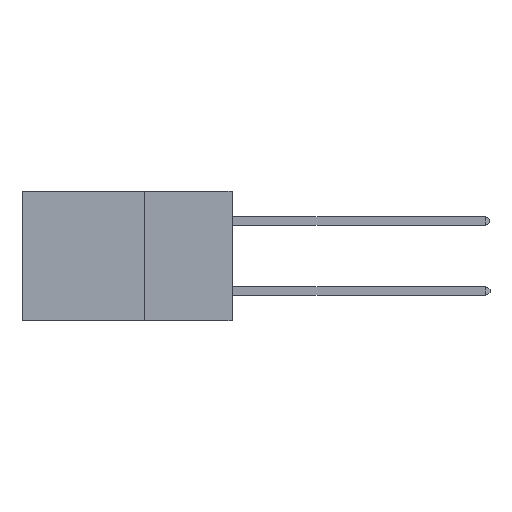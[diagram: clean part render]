
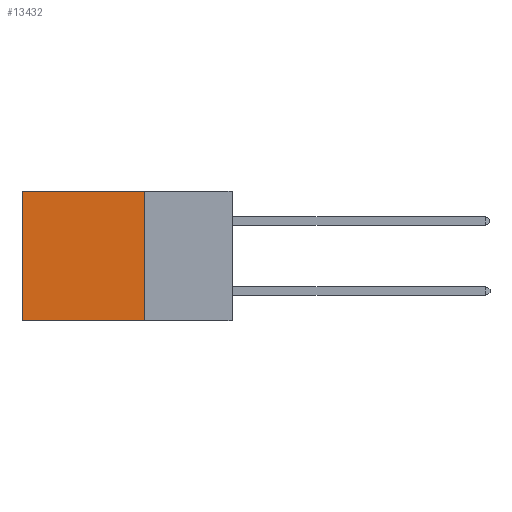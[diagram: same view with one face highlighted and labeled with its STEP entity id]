
A CAD part, left-side view. The second image highlights one B-rep face of the part: STEP entity #13432.
In plain terms, the highlighted planar face has unit normal (-1, 0, 0).
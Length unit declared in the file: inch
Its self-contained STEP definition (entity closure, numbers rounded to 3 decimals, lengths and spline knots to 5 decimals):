
#183 = CARTESIAN_POINT ( 'NONE',  ( 0.2875, 0.25, 0. ) ) ;
#424 = VECTOR ( 'NONE', #9769, 39.37008 ) ;
#2208 = CARTESIAN_POINT ( 'NONE',  ( 0.2875, 0.25, 0. ) ) ;
#2341 = VECTOR ( 'NONE', #15255, 39.37008 ) ;
#2684 = EDGE_LOOP ( 'NONE', ( #14971, #14897, #14915, #9930 ) ) ;
#2912 = EDGE_CURVE ( 'NONE', #13788, #10563, #7485, .T. ) ;
#3973 = CARTESIAN_POINT ( 'NONE',  ( 0.2875, 0.25, 0. ) ) ;
#4013 = FACE_OUTER_BOUND ( 'NONE', #2684, .T. ) ;
#4125 = CARTESIAN_POINT ( 'NONE',  ( 0.2875, 0.25, -0.37 ) ) ;
#4791 = VECTOR ( 'NONE', #8183, 39.37008 ) ;
#4951 = CARTESIAN_POINT ( 'NONE',  ( 0.2875, 0.25, -0.37 ) ) ;
#6215 = CARTESIAN_POINT ( 'NONE',  ( 0.2875, 0.25, 0. ) ) ;
#6250 = LINE ( 'NONE', #4951, #2341 ) ;
#6834 = LINE ( 'NONE', #2208, #9957 ) ;
#7485 = LINE ( 'NONE', #9855, #424 ) ;
#7552 = DIRECTION ( 'NONE',  ( 1., 0., 0. ) ) ;
#8183 = DIRECTION ( 'NONE',  ( 0., 0., -1. ) ) ;
#8412 = EDGE_CURVE ( 'NONE', #15475, #15581, #14348, .T. ) ;
#9769 = DIRECTION ( 'NONE',  ( 0., 0., -1. ) ) ;
#9855 = CARTESIAN_POINT ( 'NONE',  ( 0.2875, 0.6, 0. ) ) ;
#9929 = CARTESIAN_POINT ( 'NONE',  ( 0.2875, 0.6, -0.37 ) ) ;
#9930 = ORIENTED_EDGE ( 'NONE', *, *, #14406, .T. ) ;
#9957 = VECTOR ( 'NONE', #10134, 39.37008 ) ;
#10051 = AXIS2_PLACEMENT_3D ( 'NONE', #6215, #7552, #16421 ) ;
#10134 = DIRECTION ( 'NONE',  ( 0., 1., 0. ) ) ;
#10563 = VERTEX_POINT ( 'NONE', #9929 ) ;
#13432 = ADVANCED_FACE ( 'NONE', ( #4013 ), #14000, .F. ) ;
#13456 = EDGE_CURVE ( 'NONE', #15581, #10563, #6250, .T. ) ;
#13572 = CARTESIAN_POINT ( 'NONE',  ( 0.2875, 0.6, 0. ) ) ;
#13788 = VERTEX_POINT ( 'NONE', #13572 ) ;
#14000 = PLANE ( 'NONE',  #10051 ) ;
#14348 = LINE ( 'NONE', #183, #4791 ) ;
#14406 = EDGE_CURVE ( 'NONE', #15475, #13788, #6834, .T. ) ;
#14897 = ORIENTED_EDGE ( 'NONE', *, *, #13456, .F. ) ;
#14915 = ORIENTED_EDGE ( 'NONE', *, *, #8412, .F. ) ;
#14971 = ORIENTED_EDGE ( 'NONE', *, *, #2912, .T. ) ;
#15255 = DIRECTION ( 'NONE',  ( 0., 1., 0. ) ) ;
#15475 = VERTEX_POINT ( 'NONE', #3973 ) ;
#15581 = VERTEX_POINT ( 'NONE', #4125 ) ;
#16421 = DIRECTION ( 'NONE',  ( 0., 0., -1. ) ) ;
